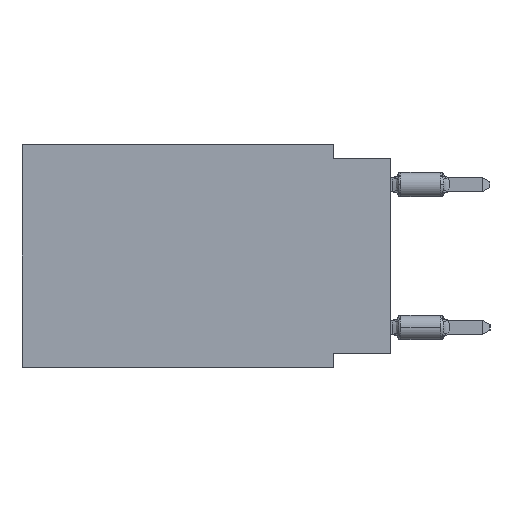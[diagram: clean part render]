
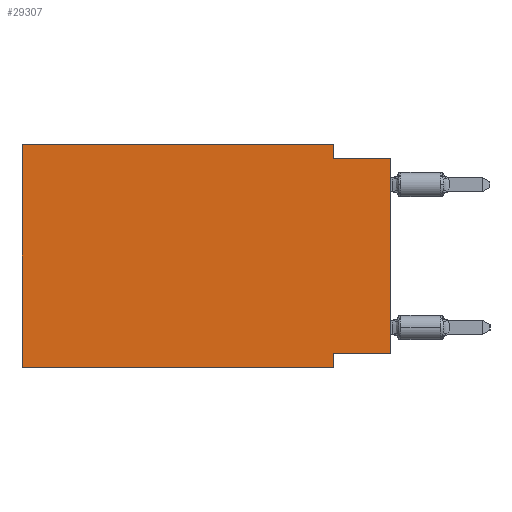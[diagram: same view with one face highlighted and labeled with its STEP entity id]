
A CAD part, left-side view. The second image highlights one B-rep face of the part: STEP entity #29307.
In plain terms, the highlighted planar face has unit normal (-1, 0, 0).
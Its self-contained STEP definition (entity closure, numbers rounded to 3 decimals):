
#86 = VERTEX_POINT ( 'NONE', #26536 ) ;
#384 = CARTESIAN_POINT ( 'NONE',  ( 0., 16.383, -9.906 ) ) ;
#462 = DIRECTION ( 'NONE',  ( 0., -1., 0. ) ) ;
#955 = VECTOR ( 'NONE', #29201, 1000. ) ;
#2972 = ORIENTED_EDGE ( 'NONE', *, *, #20392, .F. ) ;
#3521 = ORIENTED_EDGE ( 'NONE', *, *, #11847, .F. ) ;
#3865 = LINE ( 'NONE', #18346, #27322 ) ;
#5066 = VECTOR ( 'NONE', #462, 1000. ) ;
#5083 = VERTEX_POINT ( 'NONE', #21781 ) ;
#5446 = ORIENTED_EDGE ( 'NONE', *, *, #16791, .F. ) ;
#5666 = ORIENTED_EDGE ( 'NONE', *, *, #30543, .F. ) ;
#6280 = PLANE ( 'NONE',  #22578 ) ;
#6324 = LINE ( 'NONE', #16208, #22039 ) ;
#6349 = DIRECTION ( 'NONE',  ( 0., 0., 1. ) ) ;
#6368 = VECTOR ( 'NONE', #27135, 1000. ) ;
#7497 = EDGE_CURVE ( 'NONE', #21402, #9575, #16232, .T. ) ;
#7785 = CARTESIAN_POINT ( 'NONE',  ( 0., 0., -0.635 ) ) ;
#8577 = DIRECTION ( 'NONE',  ( 0., -1., 0. ) ) ;
#9429 = VECTOR ( 'NONE', #6349, 1000. ) ;
#9575 = VERTEX_POINT ( 'NONE', #24223 ) ;
#11092 = ORIENTED_EDGE ( 'NONE', *, *, #13238, .T. ) ;
#11385 = VERTEX_POINT ( 'NONE', #18554 ) ;
#11832 = DIRECTION ( 'NONE',  ( 0., 0., -1. ) ) ;
#11847 = EDGE_CURVE ( 'NONE', #86, #9575, #23926, .T. ) ;
#12024 = CARTESIAN_POINT ( 'NONE',  ( 0., 2.54, -9.906 ) ) ;
#12319 = FACE_OUTER_BOUND ( 'NONE', #16822, .T. ) ;
#12840 = LINE ( 'NONE', #12990, #5066 ) ;
#12990 = CARTESIAN_POINT ( 'NONE',  ( 0., 16.383, -9.906 ) ) ;
#13238 = EDGE_CURVE ( 'NONE', #16619, #17335, #12840, .T. ) ;
#13563 = DIRECTION ( 'NONE',  ( 0., 0., 1. ) ) ;
#14960 = CARTESIAN_POINT ( 'NONE',  ( 0., 16.383, 0. ) ) ;
#15366 = CARTESIAN_POINT ( 'NONE',  ( 0., 2.54, -9.271 ) ) ;
#15567 = ORIENTED_EDGE ( 'NONE', *, *, #29320, .F. ) ;
#16208 = CARTESIAN_POINT ( 'NONE',  ( 0., 2.54, 0. ) ) ;
#16232 = LINE ( 'NONE', #26126, #9429 ) ;
#16619 = VERTEX_POINT ( 'NONE', #384 ) ;
#16791 = EDGE_CURVE ( 'NONE', #16619, #11385, #3865, .T. ) ;
#16822 = EDGE_LOOP ( 'NONE', ( #28644, #3521, #17864, #2972, #5446, #11092, #5666, #15567 ) ) ;
#17335 = VERTEX_POINT ( 'NONE', #32158 ) ;
#17864 = ORIENTED_EDGE ( 'NONE', *, *, #30087, .F. ) ;
#18346 = CARTESIAN_POINT ( 'NONE',  ( 0., 16.383, 0. ) ) ;
#18352 = VERTEX_POINT ( 'NONE', #15366 ) ;
#18554 = CARTESIAN_POINT ( 'NONE',  ( 0., 16.383, 0. ) ) ;
#18966 = LINE ( 'NONE', #12024, #955 ) ;
#19708 = CARTESIAN_POINT ( 'NONE',  ( 0., 16.383, 0. ) ) ;
#20392 = EDGE_CURVE ( 'NONE', #11385, #5083, #25134, .T. ) ;
#21373 = CARTESIAN_POINT ( 'NONE',  ( 0., 0., -9.271 ) ) ;
#21402 = VERTEX_POINT ( 'NONE', #21373 ) ;
#21781 = CARTESIAN_POINT ( 'NONE',  ( 0., 2.54, 0. ) ) ;
#22039 = VECTOR ( 'NONE', #31237, 1000. ) ;
#22366 = DIRECTION ( 'NONE',  ( 1., 0., 0. ) ) ;
#22578 = AXIS2_PLACEMENT_3D ( 'NONE', #14960, #22366, #11832 ) ;
#23654 = VECTOR ( 'NONE', #32111, 1000. ) ;
#23926 = LINE ( 'NONE', #7785, #24278 ) ;
#24223 = CARTESIAN_POINT ( 'NONE',  ( 0., 0., -0.635 ) ) ;
#24278 = VECTOR ( 'NONE', #8577, 1000. ) ;
#24850 = LINE ( 'NONE', #27154, #23654 ) ;
#25134 = LINE ( 'NONE', #19708, #6368 ) ;
#26126 = CARTESIAN_POINT ( 'NONE',  ( 0., 0., 0. ) ) ;
#26536 = CARTESIAN_POINT ( 'NONE',  ( 0., 2.54, -0.635 ) ) ;
#27135 = DIRECTION ( 'NONE',  ( 0., -1., 0. ) ) ;
#27154 = CARTESIAN_POINT ( 'NONE',  ( 0., 0., -9.271 ) ) ;
#27322 = VECTOR ( 'NONE', #13563, 1000. ) ;
#28644 = ORIENTED_EDGE ( 'NONE', *, *, #7497, .T. ) ;
#29201 = DIRECTION ( 'NONE',  ( 0., 0., -1. ) ) ;
#29307 = ADVANCED_FACE ( 'NONE', ( #12319 ), #6280, .F. ) ;
#29320 = EDGE_CURVE ( 'NONE', #21402, #18352, #24850, .T. ) ;
#30087 = EDGE_CURVE ( 'NONE', #5083, #86, #6324, .T. ) ;
#30543 = EDGE_CURVE ( 'NONE', #18352, #17335, #18966, .T. ) ;
#31237 = DIRECTION ( 'NONE',  ( 0., 0., -1. ) ) ;
#32111 = DIRECTION ( 'NONE',  ( 0., 1., 0. ) ) ;
#32158 = CARTESIAN_POINT ( 'NONE',  ( 0., 2.54, -9.906 ) ) ;
